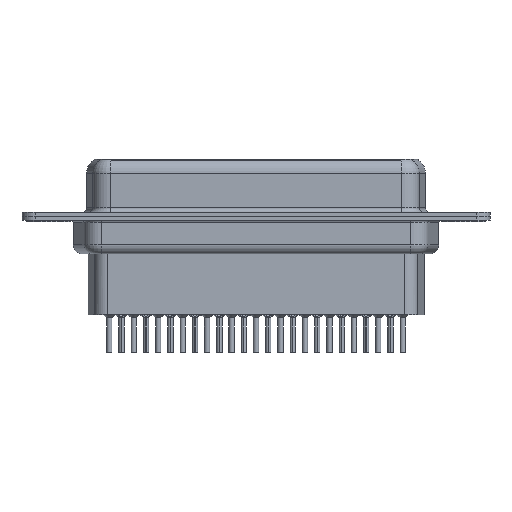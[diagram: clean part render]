
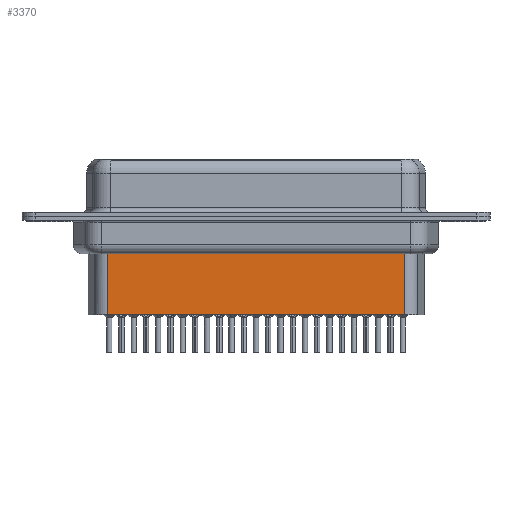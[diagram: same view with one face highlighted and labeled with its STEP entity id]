
A CAD part, front view. The second image highlights one B-rep face of the part: STEP entity #3370.
In plain terms, the highlighted planar face has unit normal (0, -1, 0).
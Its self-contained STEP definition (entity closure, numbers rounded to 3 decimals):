
#172 = CARTESIAN_POINT ( 'NONE',  ( 6.706, -3.5, -3.1 ) ) ;
#416 = DIRECTION ( 'NONE',  ( 1., 0., 0. ) ) ;
#676 = PLANE ( 'NONE',  #17221 ) ;
#727 = ORIENTED_EDGE ( 'NONE', *, *, #8528, .F. ) ;
#750 = DIRECTION ( 'NONE',  ( 0., 0., -1. ) ) ;
#975 = VECTOR ( 'NONE', #750, 1000. ) ;
#1004 = DIRECTION ( 'NONE',  ( -1., 0., 0. ) ) ;
#2395 = DIRECTION ( 'NONE',  ( 0., -1., 0. ) ) ;
#3370 = ADVANCED_FACE ( 'NONE', ( #10602 ), #676, .T. ) ;
#5612 = LINE ( 'NONE', #17379, #20363 ) ;
#7884 = VERTEX_POINT ( 'NONE', #12271 ) ;
#8528 = EDGE_CURVE ( 'NONE', #20624, #7884, #5612, .T. ) ;
#9842 = LINE ( 'NONE', #16161, #19887 ) ;
#10602 = FACE_OUTER_BOUND ( 'NONE', #16222, .T. ) ;
#12092 = CARTESIAN_POINT ( 'NONE',  ( 40.344, -3.5, -4.097 ) ) ;
#12271 = CARTESIAN_POINT ( 'NONE',  ( 40.344, -3.5, -11.15 ) ) ;
#12783 = LINE ( 'NONE', #18727, #975 ) ;
#13280 = VERTEX_POINT ( 'NONE', #15257 ) ;
#13495 = ORIENTED_EDGE ( 'NONE', *, *, #15952, .T. ) ;
#15044 = EDGE_CURVE ( 'NONE', #7884, #13280, #9842, .T. ) ;
#15257 = CARTESIAN_POINT ( 'NONE',  ( 6.706, -3.5, -11.15 ) ) ;
#15845 = VERTEX_POINT ( 'NONE', #16334 ) ;
#15952 = EDGE_CURVE ( 'NONE', #20624, #15845, #23470, .T. ) ;
#16161 = CARTESIAN_POINT ( 'NONE',  ( 6.706, -3.5, -11.15 ) ) ;
#16222 = EDGE_LOOP ( 'NONE', ( #727, #13495, #22412, #17861 ) ) ;
#16334 = CARTESIAN_POINT ( 'NONE',  ( 6.706, -3.5, -4.097 ) ) ;
#17221 = AXIS2_PLACEMENT_3D ( 'NONE', #172, #2395, #416 ) ;
#17379 = CARTESIAN_POINT ( 'NONE',  ( 40.344, -3.5, -3.1 ) ) ;
#17861 = ORIENTED_EDGE ( 'NONE', *, *, #15044, .F. ) ;
#18727 = CARTESIAN_POINT ( 'NONE',  ( 6.706, -3.5, -3.1 ) ) ;
#19887 = VECTOR ( 'NONE', #24229, 1000. ) ;
#19927 = VECTOR ( 'NONE', #1004, 1000. ) ;
#20363 = VECTOR ( 'NONE', #23601, 1000. ) ;
#20624 = VERTEX_POINT ( 'NONE', #12092 ) ;
#21440 = CARTESIAN_POINT ( 'NONE',  ( 6.459, -3.5, -4.097 ) ) ;
#22412 = ORIENTED_EDGE ( 'NONE', *, *, #25624, .T. ) ;
#23470 = LINE ( 'NONE', #21440, #19927 ) ;
#23601 = DIRECTION ( 'NONE',  ( 0., 0., -1. ) ) ;
#24229 = DIRECTION ( 'NONE',  ( -1., 0., 0. ) ) ;
#25624 = EDGE_CURVE ( 'NONE', #15845, #13280, #12783, .T. ) ;
